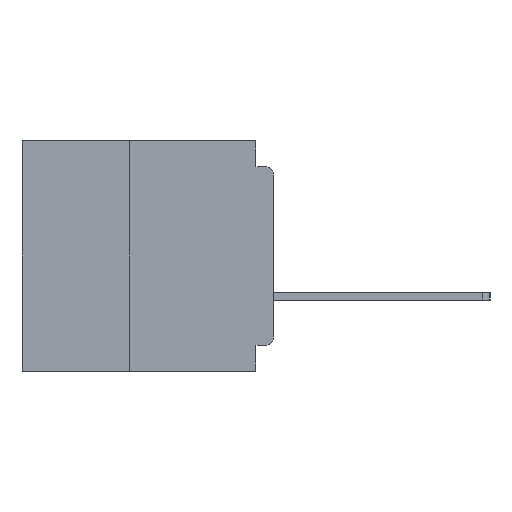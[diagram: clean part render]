
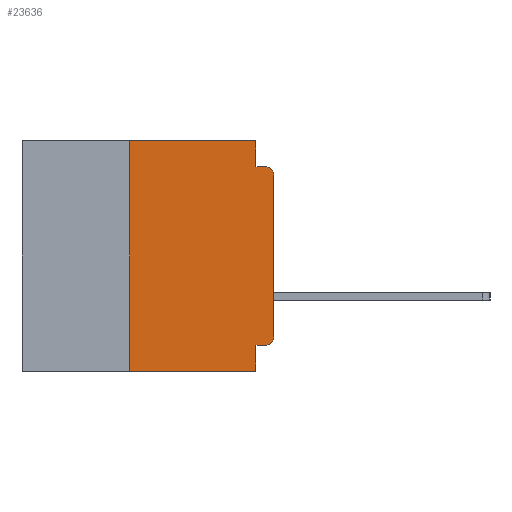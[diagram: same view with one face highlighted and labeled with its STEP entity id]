
A CAD part, left-side view. The second image highlights one B-rep face of the part: STEP entity #23636.
In plain terms, the highlighted planar face has unit normal (-1, 0, 0).
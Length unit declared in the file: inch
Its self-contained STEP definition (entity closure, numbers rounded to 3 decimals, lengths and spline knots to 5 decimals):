
#330 = VECTOR ( 'NONE', #12350, 39.37008 ) ;
#774 = DIRECTION ( 'NONE',  ( 0., 0., -1. ) ) ;
#812 = VECTOR ( 'NONE', #18118, 39.37008 ) ;
#1003 = EDGE_CURVE ( 'NONE', #46835, #36292, #13345, .T. ) ;
#1823 = VECTOR ( 'NONE', #38820, 39.37008 ) ;
#2004 = CARTESIAN_POINT ( 'NONE',  ( 0., 0.031, -0.355 ) ) ;
#2482 = DIRECTION ( 'NONE',  ( 0., 0., -1. ) ) ;
#2594 = VECTOR ( 'NONE', #13374, 39.37008 ) ;
#3942 = CIRCLE ( 'NONE', #25886, 0.015 ) ;
#4396 = CARTESIAN_POINT ( 'NONE',  ( 0., 0., -0.045 ) ) ;
#5044 = VECTOR ( 'NONE', #29146, 39.37008 ) ;
#5131 = CIRCLE ( 'NONE', #49056, 0.015 ) ;
#6195 = EDGE_CURVE ( 'NONE', #32686, #37514, #35613, .T. ) ;
#6853 = AXIS2_PLACEMENT_3D ( 'NONE', #8284, #48336, #24532 ) ;
#7404 = CARTESIAN_POINT ( 'NONE',  ( 0., 0., -0.34 ) ) ;
#8284 = CARTESIAN_POINT ( 'NONE',  ( 0., 0.437, 0. ) ) ;
#10825 = VECTOR ( 'NONE', #16450, 39.37008 ) ;
#11121 = EDGE_CURVE ( 'NONE', #41989, #46309, #43136, .T. ) ;
#11862 = ORIENTED_EDGE ( 'NONE', *, *, #44466, .F. ) ;
#12350 = DIRECTION ( 'NONE',  ( 0., -1., 0. ) ) ;
#12531 = CARTESIAN_POINT ( 'NONE',  ( 0., 0.031, -0.4 ) ) ;
#12590 = LINE ( 'NONE', #50483, #1823 ) ;
#12667 = ORIENTED_EDGE ( 'NONE', *, *, #50361, .F. ) ;
#13002 = CARTESIAN_POINT ( 'NONE',  ( 0., 0.25, 0. ) ) ;
#13075 = ORIENTED_EDGE ( 'NONE', *, *, #46931, .F. ) ;
#13345 = LINE ( 'NONE', #12531, #2594 ) ;
#13374 = DIRECTION ( 'NONE',  ( 0., 0., -1. ) ) ;
#14004 = CARTESIAN_POINT ( 'NONE',  ( 0., 0., 0. ) ) ;
#14034 = ORIENTED_EDGE ( 'NONE', *, *, #51278, .T. ) ;
#14834 = CARTESIAN_POINT ( 'NONE',  ( 0., 0.015, -0.045 ) ) ;
#16067 = CARTESIAN_POINT ( 'NONE',  ( 0., 0.25, -0.4 ) ) ;
#16181 = ORIENTED_EDGE ( 'NONE', *, *, #1003, .F. ) ;
#16411 = ORIENTED_EDGE ( 'NONE', *, *, #35692, .T. ) ;
#16450 = DIRECTION ( 'NONE',  ( 0., 1., 0. ) ) ;
#17027 = LINE ( 'NONE', #31000, #45101 ) ;
#18118 = DIRECTION ( 'NONE',  ( 0., 0., 1. ) ) ;
#19034 = CARTESIAN_POINT ( 'NONE',  ( 0., 0.031, 0. ) ) ;
#19137 = EDGE_CURVE ( 'NONE', #50357, #46835, #44053, .T. ) ;
#20465 = VECTOR ( 'NONE', #35220, 39.37008 ) ;
#20865 = CARTESIAN_POINT ( 'NONE',  ( 0., 0.437, 0. ) ) ;
#21349 = ORIENTED_EDGE ( 'NONE', *, *, #19137, .F. ) ;
#23019 = CARTESIAN_POINT ( 'NONE',  ( 0., 0.031, -0.4 ) ) ;
#23064 = ORIENTED_EDGE ( 'NONE', *, *, #11121, .F. ) ;
#23636 = ADVANCED_FACE ( 'NONE', ( #38432 ), #44355, .F. ) ;
#24532 = DIRECTION ( 'NONE',  ( 0., 0., -1. ) ) ;
#25046 = DIRECTION ( 'NONE',  ( -1., 0., 0. ) ) ;
#25886 = AXIS2_PLACEMENT_3D ( 'NONE', #48834, #25046, #774 ) ;
#26715 = DIRECTION ( 'NONE',  ( -1., 0., 0. ) ) ;
#27832 = LINE ( 'NONE', #20865, #5044 ) ;
#29146 = DIRECTION ( 'NONE',  ( 0., -1., 0. ) ) ;
#29807 = VERTEX_POINT ( 'NONE', #42888 ) ;
#31000 = CARTESIAN_POINT ( 'NONE',  ( 0., 0.25, -0.4 ) ) ;
#31162 = CARTESIAN_POINT ( 'NONE',  ( 0., 0., -0.06 ) ) ;
#32471 = CARTESIAN_POINT ( 'NONE',  ( 0., 0., -0.355 ) ) ;
#32686 = VERTEX_POINT ( 'NONE', #7404 ) ;
#32885 = VERTEX_POINT ( 'NONE', #13002 ) ;
#33012 = CARTESIAN_POINT ( 'NONE',  ( 0., 0.015, -0.355 ) ) ;
#33686 = LINE ( 'NONE', #19034, #20465 ) ;
#33987 = EDGE_LOOP ( 'NONE', ( #41715, #43607, #23064, #11862, #12667, #13075, #14034, #16181, #21349, #16411 ) ) ;
#35220 = DIRECTION ( 'NONE',  ( 0., 0., -1. ) ) ;
#35613 = LINE ( 'NONE', #14004, #812 ) ;
#35692 = EDGE_CURVE ( 'NONE', #50357, #32686, #3942, .T. ) ;
#36292 = VERTEX_POINT ( 'NONE', #23019 ) ;
#37514 = VERTEX_POINT ( 'NONE', #31162 ) ;
#38432 = FACE_OUTER_BOUND ( 'NONE', #33987, .T. ) ;
#38820 = DIRECTION ( 'NONE',  ( 0., -1., 0. ) ) ;
#38893 = CARTESIAN_POINT ( 'NONE',  ( 0., 0.031, -0.045 ) ) ;
#41715 = ORIENTED_EDGE ( 'NONE', *, *, #6195, .T. ) ;
#41989 = VERTEX_POINT ( 'NONE', #38893 ) ;
#42888 = CARTESIAN_POINT ( 'NONE',  ( 0., 0.031, 0. ) ) ;
#42928 = DIRECTION ( 'NONE',  ( 0., 0., 1. ) ) ;
#43136 = LINE ( 'NONE', #4396, #330 ) ;
#43607 = ORIENTED_EDGE ( 'NONE', *, *, #45673, .T. ) ;
#44053 = LINE ( 'NONE', #32471, #10825 ) ;
#44355 = PLANE ( 'NONE',  #6853 ) ;
#44466 = EDGE_CURVE ( 'NONE', #29807, #41989, #33686, .T. ) ;
#45101 = VECTOR ( 'NONE', #42928, 39.37008 ) ;
#45673 = EDGE_CURVE ( 'NONE', #37514, #46309, #5131, .T. ) ;
#46309 = VERTEX_POINT ( 'NONE', #14834 ) ;
#46835 = VERTEX_POINT ( 'NONE', #2004 ) ;
#46931 = EDGE_CURVE ( 'NONE', #48463, #32885, #17027, .T. ) ;
#48336 = DIRECTION ( 'NONE',  ( 1., 0., 0. ) ) ;
#48463 = VERTEX_POINT ( 'NONE', #16067 ) ;
#48834 = CARTESIAN_POINT ( 'NONE',  ( 0., 0.015, -0.34 ) ) ;
#49056 = AXIS2_PLACEMENT_3D ( 'NONE', #50440, #26715, #2482 ) ;
#50357 = VERTEX_POINT ( 'NONE', #33012 ) ;
#50361 = EDGE_CURVE ( 'NONE', #32885, #29807, #27832, .T. ) ;
#50440 = CARTESIAN_POINT ( 'NONE',  ( 0., 0.015, -0.06 ) ) ;
#50483 = CARTESIAN_POINT ( 'NONE',  ( 0., 0.437, -0.4 ) ) ;
#51278 = EDGE_CURVE ( 'NONE', #48463, #36292, #12590, .T. ) ;
